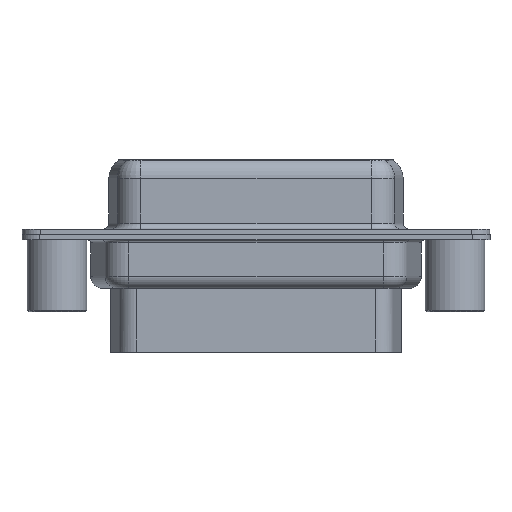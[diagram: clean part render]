
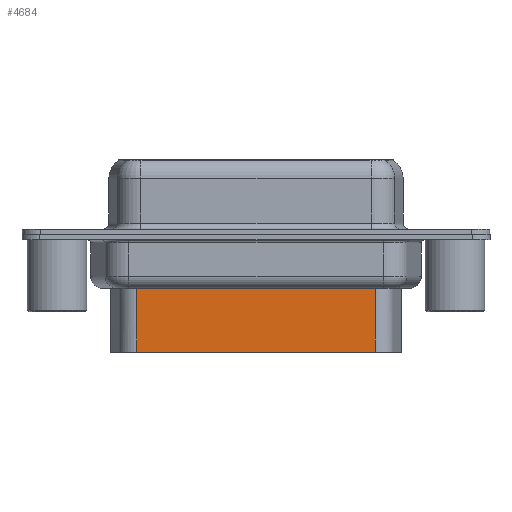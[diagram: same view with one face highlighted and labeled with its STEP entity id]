
A CAD part, front view. The second image highlights one B-rep face of the part: STEP entity #4684.
In plain terms, the highlighted planar face has unit normal (0, -1, 0).
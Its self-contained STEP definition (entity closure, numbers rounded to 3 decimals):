
#130 = EDGE_CURVE ( 'NONE', #4001, #10639, #1627, .T. ) ;
#620 = CARTESIAN_POINT ( 'NONE',  ( 6.691, -3.5, -9.85 ) ) ;
#1627 = LINE ( 'NONE', #10478, #17772 ) ;
#2024 = VECTOR ( 'NONE', #13825, 1000. ) ;
#2910 = LINE ( 'NONE', #14790, #7866 ) ;
#2962 = FACE_OUTER_BOUND ( 'NONE', #7182, .T. ) ;
#4001 = VERTEX_POINT ( 'NONE', #7192 ) ;
#4684 = ADVANCED_FACE ( 'NONE', ( #2962 ), #18053, .T. ) ;
#4981 = CARTESIAN_POINT ( 'NONE',  ( 6.691, -3.5, -9.85 ) ) ;
#6104 = DIRECTION ( 'NONE',  ( 0., -1., 0. ) ) ;
#6446 = VECTOR ( 'NONE', #10274, 1000. ) ;
#7182 = EDGE_LOOP ( 'NONE', ( #14022, #16366, #14918, #17274 ) ) ;
#7192 = CARTESIAN_POINT ( 'NONE',  ( 26.629, -3.5, -4.097 ) ) ;
#7578 = DIRECTION ( 'NONE',  ( 1., 0., 0. ) ) ;
#7866 = VECTOR ( 'NONE', #17615, 1000. ) ;
#8744 = EDGE_CURVE ( 'NONE', #10639, #10730, #2910, .T. ) ;
#9251 = AXIS2_PLACEMENT_3D ( 'NONE', #17867, #6104, #7578 ) ;
#10274 = DIRECTION ( 'NONE',  ( 0., 0., -1. ) ) ;
#10478 = CARTESIAN_POINT ( 'NONE',  ( 6.444, -3.5, -4.097 ) ) ;
#10639 = VERTEX_POINT ( 'NONE', #12207 ) ;
#10730 = VERTEX_POINT ( 'NONE', #620 ) ;
#11601 = VERTEX_POINT ( 'NONE', #14502 ) ;
#12207 = CARTESIAN_POINT ( 'NONE',  ( 6.691, -3.5, -4.097 ) ) ;
#13192 = EDGE_CURVE ( 'NONE', #4001, #11601, #16239, .T. ) ;
#13707 = DIRECTION ( 'NONE',  ( -1., 0., 0. ) ) ;
#13825 = DIRECTION ( 'NONE',  ( -1., 0., 0. ) ) ;
#14022 = ORIENTED_EDGE ( 'NONE', *, *, #13192, .F. ) ;
#14502 = CARTESIAN_POINT ( 'NONE',  ( 26.629, -3.5, -9.85 ) ) ;
#14790 = CARTESIAN_POINT ( 'NONE',  ( 6.691, -3.5, -3.1 ) ) ;
#14918 = ORIENTED_EDGE ( 'NONE', *, *, #8744, .T. ) ;
#15387 = LINE ( 'NONE', #4981, #2024 ) ;
#16239 = LINE ( 'NONE', #18962, #6446 ) ;
#16366 = ORIENTED_EDGE ( 'NONE', *, *, #130, .T. ) ;
#16775 = EDGE_CURVE ( 'NONE', #11601, #10730, #15387, .T. ) ;
#17274 = ORIENTED_EDGE ( 'NONE', *, *, #16775, .F. ) ;
#17615 = DIRECTION ( 'NONE',  ( 0., 0., -1. ) ) ;
#17772 = VECTOR ( 'NONE', #13707, 1000. ) ;
#17867 = CARTESIAN_POINT ( 'NONE',  ( 6.691, -3.5, -3.1 ) ) ;
#18053 = PLANE ( 'NONE',  #9251 ) ;
#18962 = CARTESIAN_POINT ( 'NONE',  ( 26.629, -3.5, -3.1 ) ) ;
